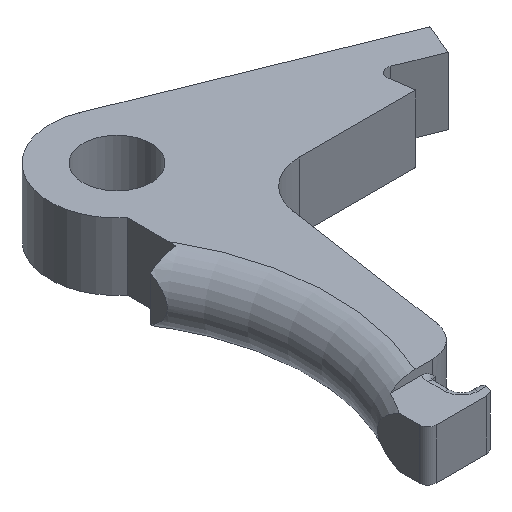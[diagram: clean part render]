
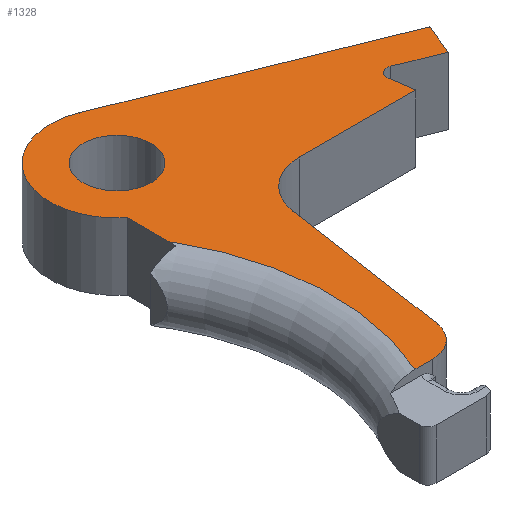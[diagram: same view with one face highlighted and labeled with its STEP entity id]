
A CAD part, isometric view. The second image highlights one B-rep face of the part: STEP entity #1328.
In plain terms, the highlighted planar face has unit normal (0, 0, 1).
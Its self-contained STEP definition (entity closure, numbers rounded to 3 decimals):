
#812=CARTESIAN_POINT('',(-3.526,-39.0,4.0));
#813=VERTEX_POINT('',#812);
#827=CARTESIAN_POINT('',(-5.,-11.188,4.0));
#828=VERTEX_POINT('',#827);
#829=CARTESIAN_POINT('',(-30.798,-26.5,4.0));
#830=DIRECTION('',(0.0,0.0,1.0));
#831=DIRECTION('',(1.0,0.0,0.0));
#832=AXIS2_PLACEMENT_3D('',#829,#830,#831);
#833=CIRCLE('',#832,30.);
#834=EDGE_CURVE('',#813,#828,#833,.T.);
#943=CARTESIAN_POINT('',(-1.443,-39.0,4.0));
#944=VERTEX_POINT('',#943);
#951=CARTESIAN_POINT('',(-1.443,-39.0,4.0));
#952=DIRECTION('',(-1.0,0.0,0.0));
#953=VECTOR('',#952,2.083);
#954=LINE('',#951,#953);
#955=EDGE_CURVE('',#944,#813,#954,.T.);
#1025=CARTESIAN_POINT('',(2.512,-35.595,4.0));
#1026=VERTEX_POINT('',#1025);
#1033=CARTESIAN_POINT('',(-1.443,-35.0,4.0));
#1034=DIRECTION('',(0.0,0.0,-1.0));
#1035=DIRECTION('',(0.652,-0.758,0.0));
#1036=AXIS2_PLACEMENT_3D('',#1033,#1034,#1035);
#1037=CIRCLE('',#1036,4.0);
#1038=EDGE_CURVE('',#1026,#944,#1037,.T.);
#1053=CARTESIAN_POINT('',(26.284,-6.305,4.0));
#1054=VERTEX_POINT('',#1053);
#1061=CARTESIAN_POINT('',(24.919,-7.372,4.0));
#1062=VERTEX_POINT('',#1061);
#1063=CARTESIAN_POINT('',(25.909,-7.232,4.0));
#1064=DIRECTION('',(0.0,0.0,1.0));
#1065=DIRECTION('',(-0.616,0.788,0.0));
#1066=AXIS2_PLACEMENT_3D('',#1063,#1064,#1065);
#1067=CIRCLE('',#1066,1.0);
#1068=EDGE_CURVE('',#1054,#1062,#1067,.T.);
#1086=CARTESIAN_POINT('',(31.168,-8.279,4.0));
#1087=VERTEX_POINT('',#1086);
#1094=CARTESIAN_POINT('',(31.168,-8.279,4.0));
#1095=DIRECTION('',(-0.927,0.375,0.0));
#1096=VECTOR('',#1095,5.268);
#1097=LINE('',#1094,#1096);
#1098=EDGE_CURVE('',#1087,#1054,#1097,.T.);
#1109=CARTESIAN_POINT('',(11.493,-10.23,4.0));
#1110=VERTEX_POINT('',#1109);
#1117=CARTESIAN_POINT('',(5.56,-15.338,4.0));
#1118=VERTEX_POINT('',#1117);
#1119=CARTESIAN_POINT('',(11.493,-16.23,4.0));
#1120=DIRECTION('',(0.0,0.0,1.0));
#1121=DIRECTION('',(-0.652,0.758,0.0));
#1122=AXIS2_PLACEMENT_3D('',#1119,#1120,#1121);
#1123=CIRCLE('',#1122,6.);
#1124=EDGE_CURVE('',#1110,#1118,#1123,.T.);
#1142=CARTESIAN_POINT('',(25.321,-10.23,4.0));
#1143=VERTEX_POINT('',#1142);
#1150=CARTESIAN_POINT('',(25.321,-10.23,4.0));
#1151=DIRECTION('',(-1.0,0.0,0.0));
#1152=VECTOR('',#1151,13.828);
#1153=LINE('',#1150,#1152);
#1154=EDGE_CURVE('',#1143,#1110,#1153,.T.);
#1167=CARTESIAN_POINT('',(4.05,0.,4.0));
#1168=VERTEX_POINT('',#1167);
#1169=CARTESIAN_POINT('',(0.0,0.0,4.0));
#1170=DIRECTION('',(0.0,0.0,-1.0));
#1171=DIRECTION('',(-1.0,0.0,0.0));
#1172=AXIS2_PLACEMENT_3D('',#1169,#1170,#1171);
#1173=CIRCLE('',#1172,4.05);
#1174=EDGE_CURVE('',#1168,#1168,#1173,.T.);
#1184=CARTESIAN_POINT('',(-5.,-6.245,4.0));
#1185=VERTEX_POINT('',#1184);
#1192=CARTESIAN_POINT('',(2.997,7.417,4.0));
#1193=VERTEX_POINT('',#1192);
#1194=CARTESIAN_POINT('',(0.0,0.0,4.0));
#1195=DIRECTION('',(0.0,0.0,-1.0));
#1196=DIRECTION('',(1.0,0.0,0.0));
#1197=AXIS2_PLACEMENT_3D('',#1194,#1195,#1196);
#1198=CIRCLE('',#1197,8.0);
#1199=EDGE_CURVE('',#1185,#1193,#1198,.T.);
#1216=CARTESIAN_POINT('',(32.667,-4.57,4.0));
#1217=VERTEX_POINT('',#1216);
#1218=CARTESIAN_POINT('',(2.997,7.417,4.0));
#1219=DIRECTION('',(0.927,-0.375,0.0));
#1220=VECTOR('',#1219,32.);
#1221=LINE('',#1218,#1220);
#1222=EDGE_CURVE('',#1193,#1217,#1221,.T.);
#1240=CARTESIAN_POINT('',(32.667,-4.57,4.0));
#1241=DIRECTION('',(-0.375,-0.927,0.0));
#1242=VECTOR('',#1241,4.);
#1243=LINE('',#1240,#1242);
#1244=EDGE_CURVE('',#1217,#1087,#1243,.T.);
#1258=CARTESIAN_POINT('',(24.919,-7.372,4.0));
#1259=DIRECTION('',(0.139,-0.99,0.0));
#1260=VECTOR('',#1259,2.887);
#1261=LINE('',#1258,#1260);
#1262=EDGE_CURVE('',#1062,#1143,#1261,.T.);
#1277=CARTESIAN_POINT('',(-5.,-11.188,4.0));
#1278=DIRECTION('',(0.0,1.0,0.0));
#1279=VECTOR('',#1278,4.943);
#1280=LINE('',#1277,#1279);
#1281=EDGE_CURVE('',#828,#1185,#1280,.T.);
#1296=CARTESIAN_POINT('',(5.56,-15.338,4.0));
#1297=DIRECTION('',(-0.149,-0.989,0.0));
#1298=VECTOR('',#1297,20.485);
#1299=LINE('',#1296,#1298);
#1300=EDGE_CURVE('',#1118,#1026,#1299,.T.);
#1305=CARTESIAN_POINT('',(-0.575,-20.956,4.0));
#1306=DIRECTION('',(0.0,0.0,1.0));
#1307=DIRECTION('',(1.0,0.0,0.0));
#1308=AXIS2_PLACEMENT_3D('',#1305,#1306,#1307);
#1309=PLANE('',#1308);
#1310=ORIENTED_EDGE('',*,*,#834,.F.);
#1311=ORIENTED_EDGE('',*,*,#955,.F.);
#1312=ORIENTED_EDGE('',*,*,#1038,.F.);
#1313=ORIENTED_EDGE('',*,*,#1300,.F.);
#1314=ORIENTED_EDGE('',*,*,#1124,.F.);
#1315=ORIENTED_EDGE('',*,*,#1154,.F.);
#1316=ORIENTED_EDGE('',*,*,#1262,.F.);
#1317=ORIENTED_EDGE('',*,*,#1068,.F.);
#1318=ORIENTED_EDGE('',*,*,#1098,.F.);
#1319=ORIENTED_EDGE('',*,*,#1244,.F.);
#1320=ORIENTED_EDGE('',*,*,#1222,.F.);
#1321=ORIENTED_EDGE('',*,*,#1199,.F.);
#1322=ORIENTED_EDGE('',*,*,#1281,.F.);
#1323=EDGE_LOOP('',(#1310,#1311,#1312,#1313,#1314,#1315,#1316,#1317,#1318,#1319,#1320,#1321,#1322));
#1324=FACE_OUTER_BOUND('',#1323,.T.);
#1325=ORIENTED_EDGE('',*,*,#1174,.T.);
#1326=EDGE_LOOP('',(#1325));
#1327=FACE_BOUND('',#1326,.T.);
#1328=ADVANCED_FACE('',(#1324,#1327),#1309,.T.);
